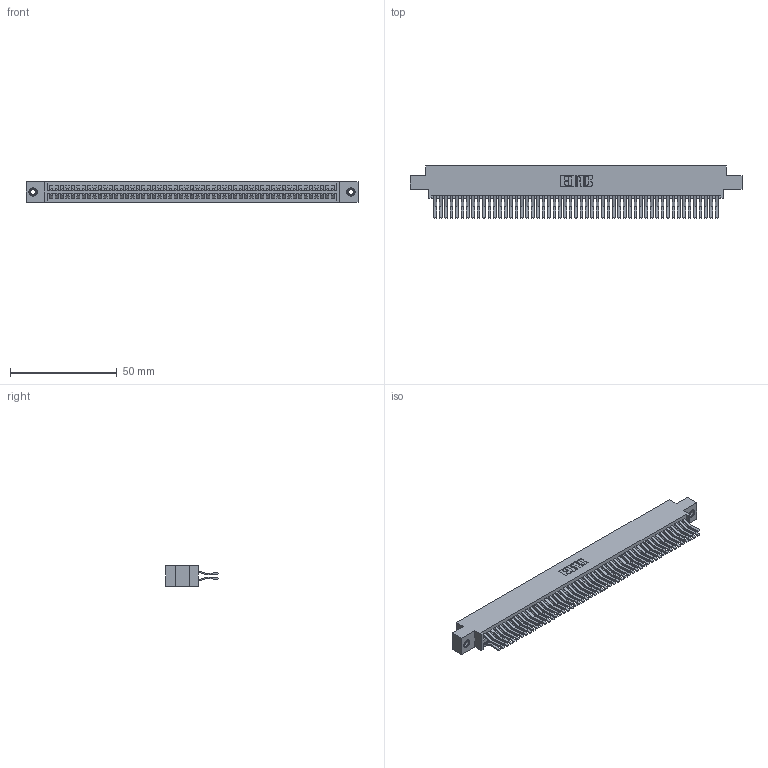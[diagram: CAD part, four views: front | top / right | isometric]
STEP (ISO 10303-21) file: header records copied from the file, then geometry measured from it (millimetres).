
FILE_DESCRIPTION (( 'STEP AP203' ), '1' );
FILE_NAME ('395-106-560-808.STEP', '2018-11-30T19:39:36', ( '' ), ( '' ), 'SwSTEP 2.0', 'SolidWorks 2016', '' );
FILE_SCHEMA (( 'CONFIG_CONTROL_DESIGN' ));
Length unit declared in the file: inch
Products named in the file (4): 345-292-001_560 Tail; 345-250-001_345-250-003-102; 395-106-560-808; 345 Part_0.170 Offset - 0.156 Dia-TI
Assembly tree (109 placements, depth 2):
  395-106-560-808
    345 Part_0.170 Offset - 0.156 Dia-TI
    345-292-001_560 Tail  x106
    345-250-001_345-250-003-102  x2
Bounding box: 155.83 x 24.45 x 9.4 mm (x, y, z)
Volume: 15814.4 mm3; surface area: 25533.2 mm2
Topology: 109 solids, 109 shells, 5702 faces, 16919 edges, 11130 vertices
Faces by surface type: plane 3614, cylinder 2072, cone 12, torus 4
Entity records: 41510 total; most frequent: CARTESIAN_POINT 6931, ORIENTED_EDGE 6858, DIRECTION 6127, EDGE_CURVE 3429, LINE 3061, VECTOR 3061, VERTEX_POINT 2280, AXIS2_PLACEMENT_3D 1533
